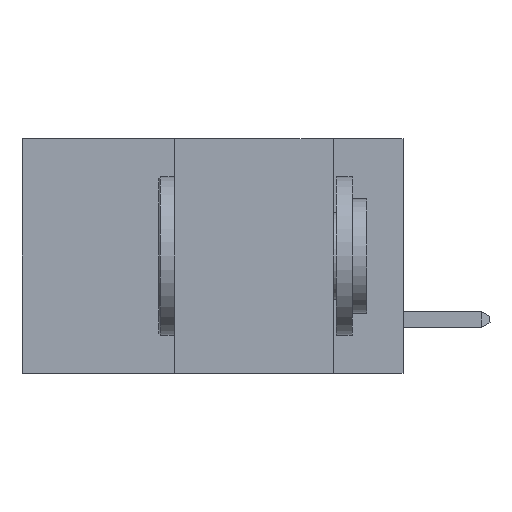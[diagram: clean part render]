
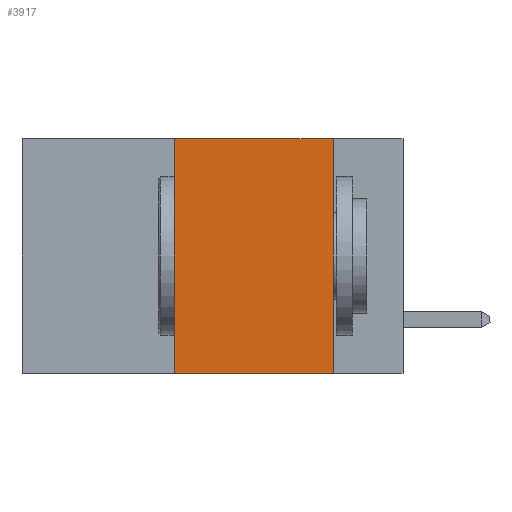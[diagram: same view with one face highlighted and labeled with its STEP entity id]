
A CAD part, left-side view. The second image highlights one B-rep face of the part: STEP entity #3917.
In plain terms, the highlighted planar face has unit normal (-1, 0, 0).
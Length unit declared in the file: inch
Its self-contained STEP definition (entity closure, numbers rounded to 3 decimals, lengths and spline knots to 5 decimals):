
#468 = EDGE_CURVE ( 'NONE', #11454, #21837, #22303, .T. ) ;
#1846 = CARTESIAN_POINT ( 'NONE',  ( 0., 0.36, 0. ) ) ;
#1911 = EDGE_CURVE ( 'NONE', #4975, #14636, #8330, .T. ) ;
#1995 = LINE ( 'NONE', #2130, #16890 ) ;
#2130 = CARTESIAN_POINT ( 'NONE',  ( 0., 0.11, 0. ) ) ;
#2688 = VECTOR ( 'NONE', #8306, 39.37008 ) ;
#3350 = DIRECTION ( 'NONE',  ( 0., 0., -1. ) ) ;
#3389 = DIRECTION ( 'NONE',  ( 1., 0., 0. ) ) ;
#3506 = CARTESIAN_POINT ( 'NONE',  ( 0., 0.6, 0. ) ) ;
#3917 = ADVANCED_FACE ( 'NONE', ( #18667 ), #4045, .F. ) ;
#4045 = PLANE ( 'NONE',  #14529 ) ;
#4270 = DIRECTION ( 'NONE',  ( 0., 0., -1. ) ) ;
#4975 = VERTEX_POINT ( 'NONE', #24897 ) ;
#5258 = CARTESIAN_POINT ( 'NONE',  ( 0., 0.11, -0.37 ) ) ;
#5422 = CARTESIAN_POINT ( 'NONE',  ( 0., 0.36, 0. ) ) ;
#6212 = CARTESIAN_POINT ( 'NONE',  ( 0., 0.6, 0. ) ) ;
#7658 = DIRECTION ( 'NONE',  ( 0., -1., 0. ) ) ;
#8263 = CARTESIAN_POINT ( 'NONE',  ( 0., 0.6, -0.37 ) ) ;
#8306 = DIRECTION ( 'NONE',  ( 0., -1., 0. ) ) ;
#8330 = LINE ( 'NONE', #8263, #2688 ) ;
#11357 = ORIENTED_EDGE ( 'NONE', *, *, #24359, .F. ) ;
#11454 = VERTEX_POINT ( 'NONE', #1846 ) ;
#13092 = ORIENTED_EDGE ( 'NONE', *, *, #1911, .T. ) ;
#13355 = EDGE_CURVE ( 'NONE', #4975, #11454, #16714, .T. ) ;
#14080 = ORIENTED_EDGE ( 'NONE', *, *, #13355, .F. ) ;
#14529 = AXIS2_PLACEMENT_3D ( 'NONE', #3506, #3389, #3350 ) ;
#14636 = VERTEX_POINT ( 'NONE', #5258 ) ;
#16714 = LINE ( 'NONE', #5422, #21421 ) ;
#16890 = VECTOR ( 'NONE', #4270, 39.37008 ) ;
#18366 = CARTESIAN_POINT ( 'NONE',  ( 0., 0.11, 0. ) ) ;
#18667 = FACE_OUTER_BOUND ( 'NONE', #20777, .T. ) ;
#18913 = ORIENTED_EDGE ( 'NONE', *, *, #468, .F. ) ;
#20777 = EDGE_LOOP ( 'NONE', ( #11357, #18913, #14080, #13092 ) ) ;
#21421 = VECTOR ( 'NONE', #22082, 39.37008 ) ;
#21670 = VECTOR ( 'NONE', #7658, 39.37008 ) ;
#21837 = VERTEX_POINT ( 'NONE', #18366 ) ;
#22082 = DIRECTION ( 'NONE',  ( 0., 0., 1. ) ) ;
#22303 = LINE ( 'NONE', #6212, #21670 ) ;
#24359 = EDGE_CURVE ( 'NONE', #21837, #14636, #1995, .T. ) ;
#24897 = CARTESIAN_POINT ( 'NONE',  ( 0., 0.36, -0.37 ) ) ;
